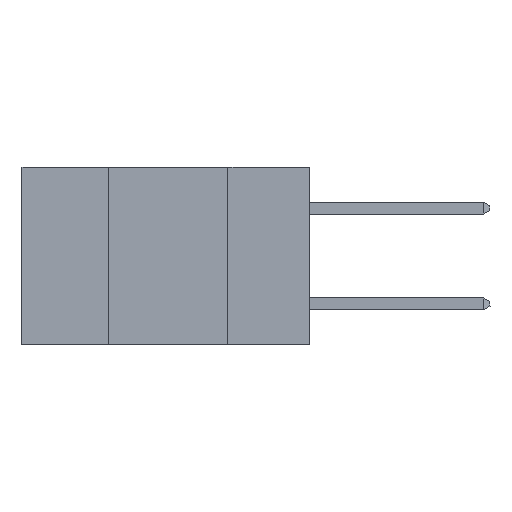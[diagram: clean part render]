
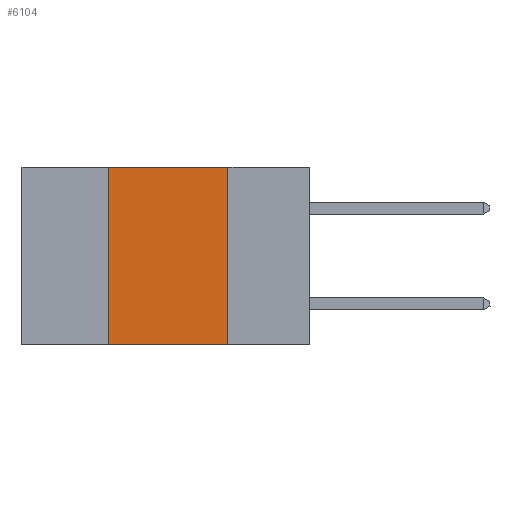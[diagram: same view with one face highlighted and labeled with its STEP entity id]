
A CAD part, left-side view. The second image highlights one B-rep face of the part: STEP entity #6104.
In plain terms, the highlighted planar face has unit normal (-1, 0, 0).
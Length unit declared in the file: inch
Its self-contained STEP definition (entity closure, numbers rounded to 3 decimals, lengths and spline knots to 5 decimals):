
#241 = VECTOR ( 'NONE', #19242, 39.37008 ) ;
#1161 = CARTESIAN_POINT ( 'NONE',  ( 0., 0.17, -0.37 ) ) ;
#1289 = VERTEX_POINT ( 'NONE', #18278 ) ;
#1827 = ORIENTED_EDGE ( 'NONE', *, *, #13428, .T. ) ;
#2514 = ORIENTED_EDGE ( 'NONE', *, *, #3063, .F. ) ;
#2950 = PLANE ( 'NONE',  #8928 ) ;
#3042 = DIRECTION ( 'NONE',  ( 0., -1., 0. ) ) ;
#3063 = EDGE_CURVE ( 'NONE', #1289, #5455, #17717, .T. ) ;
#4081 = CARTESIAN_POINT ( 'NONE',  ( 0., 0.6, -0.37 ) ) ;
#4322 = LINE ( 'NONE', #17735, #241 ) ;
#4364 = DIRECTION ( 'NONE',  ( 0., 0., -1. ) ) ;
#4422 = CARTESIAN_POINT ( 'NONE',  ( 0., 0.6, 0. ) ) ;
#5455 = VERTEX_POINT ( 'NONE', #1161 ) ;
#5492 = DIRECTION ( 'NONE',  ( 0., -1., 0. ) ) ;
#6104 = ADVANCED_FACE ( 'NONE', ( #8657 ), #2950, .F. ) ;
#6317 = VECTOR ( 'NONE', #4364, 39.37008 ) ;
#8373 = ORIENTED_EDGE ( 'NONE', *, *, #14447, .F. ) ;
#8657 = FACE_OUTER_BOUND ( 'NONE', #9689, .T. ) ;
#8928 = AXIS2_PLACEMENT_3D ( 'NONE', #4422, #19281, #10533 ) ;
#9689 = EDGE_LOOP ( 'NONE', ( #2514, #14425, #8373, #1827 ) ) ;
#10055 = LINE ( 'NONE', #4081, #17357 ) ;
#10533 = DIRECTION ( 'NONE',  ( 0., 0., -1. ) ) ;
#10556 = CARTESIAN_POINT ( 'NONE',  ( 0., 0.6, 0. ) ) ;
#11791 = EDGE_CURVE ( 'NONE', #17351, #1289, #16963, .T. ) ;
#13428 = EDGE_CURVE ( 'NONE', #14140, #5455, #10055, .T. ) ;
#13489 = CARTESIAN_POINT ( 'NONE',  ( 0., 0.42, 0. ) ) ;
#14140 = VERTEX_POINT ( 'NONE', #15665 ) ;
#14425 = ORIENTED_EDGE ( 'NONE', *, *, #11791, .F. ) ;
#14447 = EDGE_CURVE ( 'NONE', #14140, #17351, #4322, .T. ) ;
#15665 = CARTESIAN_POINT ( 'NONE',  ( 0., 0.42, -0.37 ) ) ;
#16512 = VECTOR ( 'NONE', #3042, 39.37008 ) ;
#16963 = LINE ( 'NONE', #10556, #16512 ) ;
#17351 = VERTEX_POINT ( 'NONE', #13489 ) ;
#17357 = VECTOR ( 'NONE', #5492, 39.37008 ) ;
#17705 = CARTESIAN_POINT ( 'NONE',  ( 0., 0.17, 0. ) ) ;
#17717 = LINE ( 'NONE', #17705, #6317 ) ;
#17735 = CARTESIAN_POINT ( 'NONE',  ( 0., 0.42, 0. ) ) ;
#18278 = CARTESIAN_POINT ( 'NONE',  ( 0., 0.17, 0. ) ) ;
#19242 = DIRECTION ( 'NONE',  ( 0., 0., 1. ) ) ;
#19281 = DIRECTION ( 'NONE',  ( 1., 0., 0. ) ) ;
